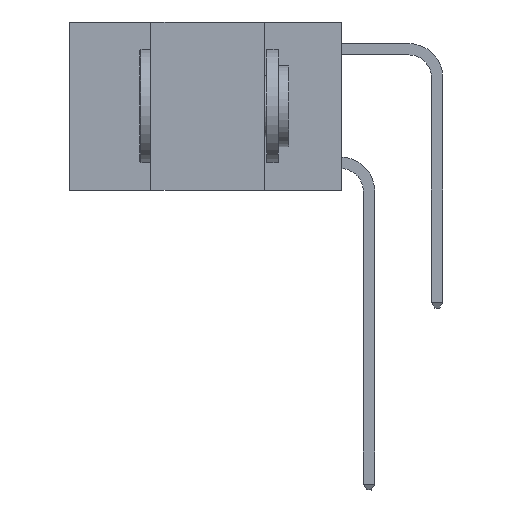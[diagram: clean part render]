
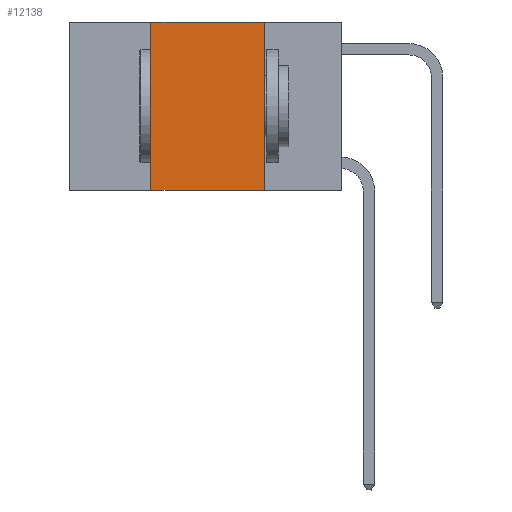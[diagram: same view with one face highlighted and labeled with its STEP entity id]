
A CAD part, left-side view. The second image highlights one B-rep face of the part: STEP entity #12138.
In plain terms, the highlighted planar face has unit normal (-1, 0, 0).
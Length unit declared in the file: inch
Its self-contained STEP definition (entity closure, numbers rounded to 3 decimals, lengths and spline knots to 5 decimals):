
#833 = PLANE ( 'NONE',  #7158 ) ;
#901 = FACE_OUTER_BOUND ( 'NONE', #1459, .T. ) ;
#1208 = ORIENTED_EDGE ( 'NONE', *, *, #1658, .F. ) ;
#1277 = DIRECTION ( 'NONE',  ( 0., -1., 0. ) ) ;
#1427 = VECTOR ( 'NONE', #14969, 39.37008 ) ;
#1459 = EDGE_LOOP ( 'NONE', ( #7602, #14280, #1208, #13054 ) ) ;
#1658 = EDGE_CURVE ( 'NONE', #6236, #11550, #2634, .T. ) ;
#1903 = EDGE_CURVE ( 'NONE', #6236, #15031, #14002, .T. ) ;
#2469 = LINE ( 'NONE', #12319, #8369 ) ;
#2634 = LINE ( 'NONE', #6123, #8126 ) ;
#2734 = VECTOR ( 'NONE', #13746, 39.37008 ) ;
#3162 = CARTESIAN_POINT ( 'NONE',  ( 0., 0.6, 0. ) ) ;
#3235 = EDGE_CURVE ( 'NONE', #9212, #15031, #7954, .T. ) ;
#3921 = EDGE_CURVE ( 'NONE', #11550, #9212, #2469, .T. ) ;
#4329 = CARTESIAN_POINT ( 'NONE',  ( 0., 0.17, 0. ) ) ;
#6123 = CARTESIAN_POINT ( 'NONE',  ( 0., 0.42, 0. ) ) ;
#6236 = VERTEX_POINT ( 'NONE', #14159 ) ;
#6817 = DIRECTION ( 'NONE',  ( 0., 0., -1. ) ) ;
#7158 = AXIS2_PLACEMENT_3D ( 'NONE', #3162, #13002, #6817 ) ;
#7602 = ORIENTED_EDGE ( 'NONE', *, *, #3235, .F. ) ;
#7954 = LINE ( 'NONE', #4329, #2734 ) ;
#8126 = VECTOR ( 'NONE', #12397, 39.37008 ) ;
#8369 = VECTOR ( 'NONE', #1277, 39.37008 ) ;
#9212 = VERTEX_POINT ( 'NONE', #13263 ) ;
#9632 = CARTESIAN_POINT ( 'NONE',  ( 0., 0.17, -0.37 ) ) ;
#11550 = VERTEX_POINT ( 'NONE', #13747 ) ;
#12138 = ADVANCED_FACE ( 'NONE', ( #901 ), #833, .F. ) ;
#12319 = CARTESIAN_POINT ( 'NONE',  ( 0., 0.6, 0. ) ) ;
#12397 = DIRECTION ( 'NONE',  ( 0., 0., 1. ) ) ;
#12642 = CARTESIAN_POINT ( 'NONE',  ( 0., 0.6, -0.37 ) ) ;
#13002 = DIRECTION ( 'NONE',  ( 1., 0., 0. ) ) ;
#13054 = ORIENTED_EDGE ( 'NONE', *, *, #1903, .T. ) ;
#13263 = CARTESIAN_POINT ( 'NONE',  ( 0., 0.17, 0. ) ) ;
#13746 = DIRECTION ( 'NONE',  ( 0., 0., -1. ) ) ;
#13747 = CARTESIAN_POINT ( 'NONE',  ( 0., 0.42, 0. ) ) ;
#14002 = LINE ( 'NONE', #12642, #1427 ) ;
#14159 = CARTESIAN_POINT ( 'NONE',  ( 0., 0.42, -0.37 ) ) ;
#14280 = ORIENTED_EDGE ( 'NONE', *, *, #3921, .F. ) ;
#14969 = DIRECTION ( 'NONE',  ( 0., -1., 0. ) ) ;
#15031 = VERTEX_POINT ( 'NONE', #9632 ) ;
